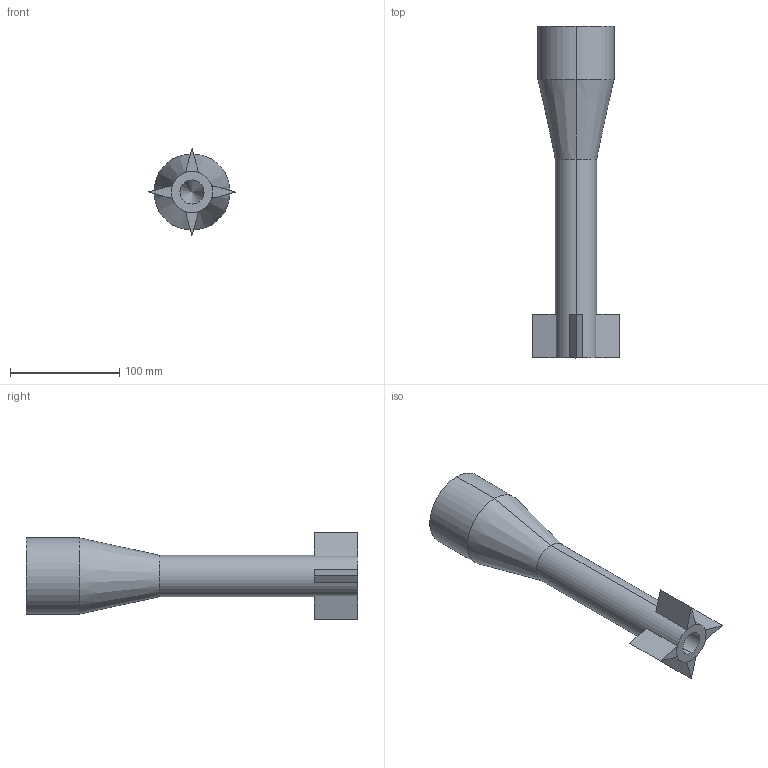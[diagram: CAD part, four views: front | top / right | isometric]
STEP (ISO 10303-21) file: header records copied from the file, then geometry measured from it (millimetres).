
FILE_DESCRIPTION (( 'STEP AP214' ), '1' );
FILE_NAME ('base.STEP', '2014-04-06T05:14:18', ( 'eric' ), ( '' ), 'SwSTEP 2.0', 'SolidWorks 2012', '' );
FILE_SCHEMA (( 'AUTOMOTIVE_DESIGN' ));
Length unit declared in the file: millimetre
Products named in the file (1): base
Bounding box: 80 x 304 x 80 mm (x, y, z)
Volume: 245843.7 mm3; surface area: 89549.6 mm2
Topology: 5 solids, 5 shells, 43 faces, 83 edges, 51 vertices
Faces by surface type: plane 20, cylinder 17, cone 6
Entity records: 1169 total; most frequent: DIRECTION 203, CARTESIAN_POINT 176, ORIENTED_EDGE 162, EDGE_CURVE 81, AXIS2_PLACEMENT_3D 78, VERTEX_POINT 51, LINE 47, VECTOR 47
